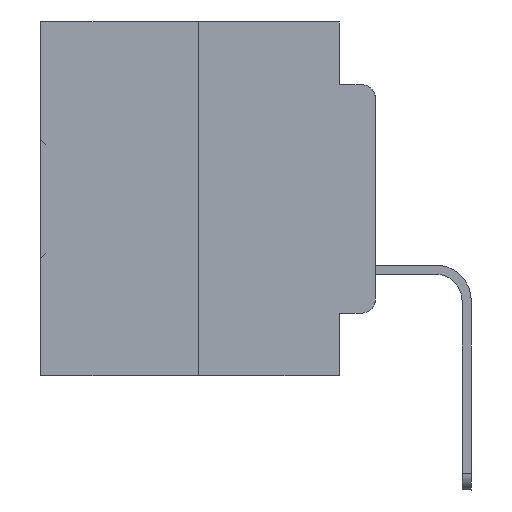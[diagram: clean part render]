
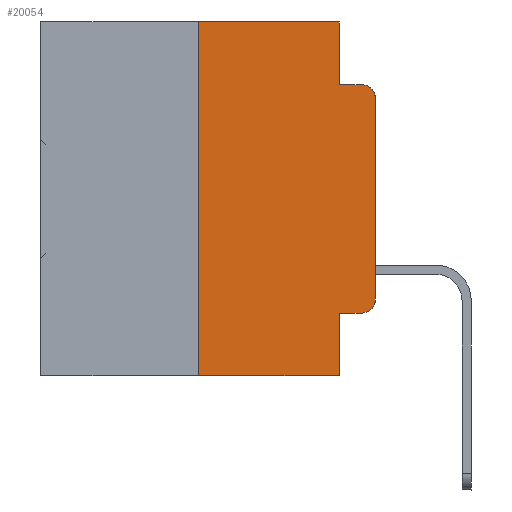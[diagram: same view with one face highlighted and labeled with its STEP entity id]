
A CAD part, left-side view. The second image highlights one B-rep face of the part: STEP entity #20054.
In plain terms, the highlighted planar face has unit normal (-1, 0, 0).
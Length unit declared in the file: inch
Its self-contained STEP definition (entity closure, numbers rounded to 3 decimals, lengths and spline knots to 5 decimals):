
#321 = ORIENTED_EDGE ( 'NONE', *, *, #20945, .F. ) ;
#1396 = EDGE_LOOP ( 'NONE', ( #8482, #9585, #12731, #321, #2469, #7651, #31808, #21415, #22508, #5339 ) ) ;
#2121 = VERTEX_POINT ( 'NONE', #7090 ) ;
#2440 = EDGE_CURVE ( 'NONE', #24323, #15689, #9093, .T. ) ;
#2469 = ORIENTED_EDGE ( 'NONE', *, *, #27839, .F. ) ;
#2781 = DIRECTION ( 'NONE',  ( 0., 0., 1. ) ) ;
#2974 = CARTESIAN_POINT ( 'NONE',  ( 0., 0.02, -0.0885 ) ) ;
#3025 = DIRECTION ( 'NONE',  ( 0., -1., 0. ) ) ;
#3574 = CARTESIAN_POINT ( 'NONE',  ( 0., 0., 0. ) ) ;
#4593 = DIRECTION ( 'NONE',  ( 0., -1., 0. ) ) ;
#5271 = VERTEX_POINT ( 'NONE', #24123 ) ;
#5339 = ORIENTED_EDGE ( 'NONE', *, *, #26811, .T. ) ;
#5401 = LINE ( 'NONE', #23147, #18894 ) ;
#6924 = VERTEX_POINT ( 'NONE', #30045 ) ;
#6948 = VECTOR ( 'NONE', #4593, 39.37008 ) ;
#7090 = CARTESIAN_POINT ( 'NONE',  ( 0., 0.051, -0.5 ) ) ;
#7122 = CARTESIAN_POINT ( 'NONE',  ( 0., 0.051, -0.0885 ) ) ;
#7200 = CARTESIAN_POINT ( 'NONE',  ( 0., 0., -0.1085 ) ) ;
#7221 = CARTESIAN_POINT ( 'NONE',  ( 0., 0.051, 0. ) ) ;
#7385 = CARTESIAN_POINT ( 'NONE',  ( 0., 0.25, -0.5 ) ) ;
#7651 = ORIENTED_EDGE ( 'NONE', *, *, #23028, .F. ) ;
#7666 = EDGE_CURVE ( 'NONE', #7945, #2121, #12618, .T. ) ;
#7945 = VERTEX_POINT ( 'NONE', #8079 ) ;
#8079 = CARTESIAN_POINT ( 'NONE',  ( 0., 0.051, -0.4115 ) ) ;
#8482 = ORIENTED_EDGE ( 'NONE', *, *, #2440, .T. ) ;
#9093 = LINE ( 'NONE', #3574, #19309 ) ;
#9391 = VERTEX_POINT ( 'NONE', #7122 ) ;
#9585 = ORIENTED_EDGE ( 'NONE', *, *, #28055, .T. ) ;
#10364 = LINE ( 'NONE', #29029, #16526 ) ;
#10758 = EDGE_CURVE ( 'NONE', #9391, #21744, #10364, .T. ) ;
#11778 = DIRECTION ( 'NONE',  ( 0., 0., 1. ) ) ;
#12245 = CARTESIAN_POINT ( 'NONE',  ( 0., 0.473, 0. ) ) ;
#12618 = LINE ( 'NONE', #20233, #29057 ) ;
#12731 = ORIENTED_EDGE ( 'NONE', *, *, #10758, .F. ) ;
#13277 = EDGE_CURVE ( 'NONE', #13905, #2121, #22534, .T. ) ;
#13905 = VERTEX_POINT ( 'NONE', #7385 ) ;
#14132 = AXIS2_PLACEMENT_3D ( 'NONE', #25506, #33462, #23767 ) ;
#14674 = DIRECTION ( 'NONE',  ( 1., 0., 0. ) ) ;
#15689 = VERTEX_POINT ( 'NONE', #7200 ) ;
#16006 = VECTOR ( 'NONE', #25340, 39.37008 ) ;
#16114 = AXIS2_PLACEMENT_3D ( 'NONE', #24283, #32139, #16457 ) ;
#16272 = CARTESIAN_POINT ( 'NONE',  ( 0., 0.25, 0. ) ) ;
#16457 = DIRECTION ( 'NONE',  ( 0., 0., -1. ) ) ;
#16526 = VECTOR ( 'NONE', #3025, 39.37008 ) ;
#17267 = LINE ( 'NONE', #16272, #26298 ) ;
#17940 = DIRECTION ( 'NONE',  ( 0., -1., 0. ) ) ;
#18564 = LINE ( 'NONE', #27647, #26796 ) ;
#18894 = VECTOR ( 'NONE', #17940, 39.37008 ) ;
#18959 = LINE ( 'NONE', #22693, #16006 ) ;
#19309 = VECTOR ( 'NONE', #11778, 39.37008 ) ;
#19606 = PLANE ( 'NONE',  #21979 ) ;
#20054 = ADVANCED_FACE ( 'NONE', ( #24345 ), #19606, .F. ) ;
#20233 = CARTESIAN_POINT ( 'NONE',  ( 0., 0.051, 0. ) ) ;
#20945 = EDGE_CURVE ( 'NONE', #23409, #9391, #18564, .T. ) ;
#21415 = ORIENTED_EDGE ( 'NONE', *, *, #7666, .F. ) ;
#21744 = VERTEX_POINT ( 'NONE', #2974 ) ;
#21979 = AXIS2_PLACEMENT_3D ( 'NONE', #12245, #14674, #33196 ) ;
#22508 = ORIENTED_EDGE ( 'NONE', *, *, #26018, .T. ) ;
#22534 = LINE ( 'NONE', #27953, #6948 ) ;
#22693 = CARTESIAN_POINT ( 'NONE',  ( 0., 0.051, -0.4115 ) ) ;
#23028 = EDGE_CURVE ( 'NONE', #13905, #5271, #17267, .T. ) ;
#23147 = CARTESIAN_POINT ( 'NONE',  ( 0., 0.473, 0. ) ) ;
#23409 = VERTEX_POINT ( 'NONE', #7221 ) ;
#23767 = DIRECTION ( 'NONE',  ( 0., 0., -1. ) ) ;
#24123 = CARTESIAN_POINT ( 'NONE',  ( 0., 0.25, 0. ) ) ;
#24283 = CARTESIAN_POINT ( 'NONE',  ( 0., 0.02, -0.1085 ) ) ;
#24323 = VERTEX_POINT ( 'NONE', #33779 ) ;
#24345 = FACE_OUTER_BOUND ( 'NONE', #1396, .T. ) ;
#25152 = CIRCLE ( 'NONE', #14132, 0.02 ) ;
#25340 = DIRECTION ( 'NONE',  ( 0., -1., 0. ) ) ;
#25506 = CARTESIAN_POINT ( 'NONE',  ( 0., 0.02, -0.3915 ) ) ;
#26018 = EDGE_CURVE ( 'NONE', #7945, #6924, #18959, .T. ) ;
#26298 = VECTOR ( 'NONE', #2781, 39.37008 ) ;
#26796 = VECTOR ( 'NONE', #27760, 39.37008 ) ;
#26811 = EDGE_CURVE ( 'NONE', #6924, #24323, #25152, .T. ) ;
#27647 = CARTESIAN_POINT ( 'NONE',  ( 0., 0.051, 0. ) ) ;
#27760 = DIRECTION ( 'NONE',  ( 0., 0., -1. ) ) ;
#27839 = EDGE_CURVE ( 'NONE', #5271, #23409, #5401, .T. ) ;
#27953 = CARTESIAN_POINT ( 'NONE',  ( 0., 0.473, -0.5 ) ) ;
#28055 = EDGE_CURVE ( 'NONE', #15689, #21744, #29562, .T. ) ;
#29029 = CARTESIAN_POINT ( 'NONE',  ( 0., 0.051, -0.0885 ) ) ;
#29057 = VECTOR ( 'NONE', #32946, 39.37008 ) ;
#29562 = CIRCLE ( 'NONE', #16114, 0.02 ) ;
#30045 = CARTESIAN_POINT ( 'NONE',  ( 0., 0.02, -0.4115 ) ) ;
#31808 = ORIENTED_EDGE ( 'NONE', *, *, #13277, .T. ) ;
#32139 = DIRECTION ( 'NONE',  ( -1., 0., 0. ) ) ;
#32946 = DIRECTION ( 'NONE',  ( 0., 0., -1. ) ) ;
#33196 = DIRECTION ( 'NONE',  ( 0., 0., -1. ) ) ;
#33462 = DIRECTION ( 'NONE',  ( -1., 0., 0. ) ) ;
#33779 = CARTESIAN_POINT ( 'NONE',  ( 0., 0., -0.3915 ) ) ;
